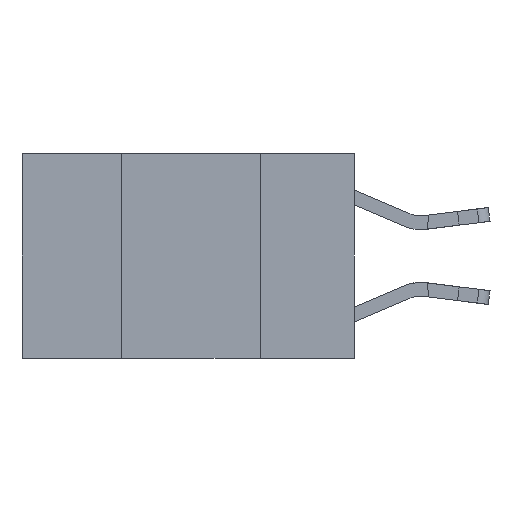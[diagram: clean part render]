
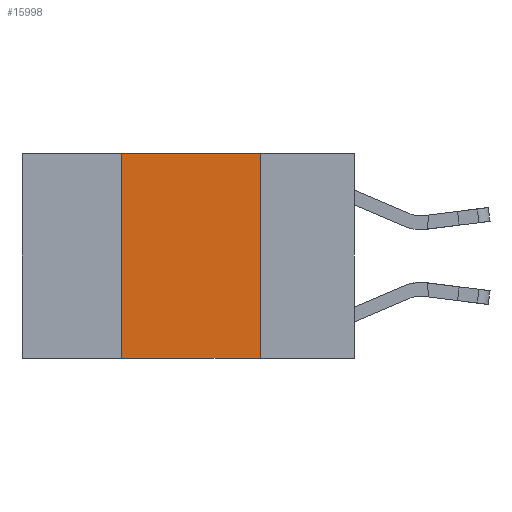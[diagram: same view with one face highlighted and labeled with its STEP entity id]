
A CAD part, left-side view. The second image highlights one B-rep face of the part: STEP entity #15998.
In plain terms, the highlighted planar face has unit normal (-1, 0, 0).
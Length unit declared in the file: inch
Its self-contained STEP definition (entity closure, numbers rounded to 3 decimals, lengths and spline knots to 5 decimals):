
#280 = EDGE_CURVE ( 'NONE', #7859, #16277, #9173, .T. ) ;
#2634 = CARTESIAN_POINT ( 'NONE',  ( 0., 0.42, -0.37 ) ) ;
#3594 = LINE ( 'NONE', #17894, #19074 ) ;
#4915 = LINE ( 'NONE', #13731, #21497 ) ;
#5844 = CARTESIAN_POINT ( 'NONE',  ( 0., 0.6, -0.37 ) ) ;
#5894 = EDGE_CURVE ( 'NONE', #19968, #14642, #3594, .T. ) ;
#7270 = FACE_OUTER_BOUND ( 'NONE', #21542, .T. ) ;
#7387 = ORIENTED_EDGE ( 'NONE', *, *, #16725, .F. ) ;
#7682 = DIRECTION ( 'NONE',  ( 0., -1., 0. ) ) ;
#7859 = VERTEX_POINT ( 'NONE', #2634 ) ;
#8364 = ORIENTED_EDGE ( 'NONE', *, *, #5894, .F. ) ;
#8982 = CARTESIAN_POINT ( 'NONE',  ( 0., 0.17, 0. ) ) ;
#9112 = VECTOR ( 'NONE', #17543, 39.37008 ) ;
#9173 = LINE ( 'NONE', #5844, #22106 ) ;
#10591 = DIRECTION ( 'NONE',  ( 1., 0., 0. ) ) ;
#11042 = DIRECTION ( 'NONE',  ( 0., 0., -1. ) ) ;
#11798 = DIRECTION ( 'NONE',  ( 0., 0., -1. ) ) ;
#13731 = CARTESIAN_POINT ( 'NONE',  ( 0., 0.17, 0. ) ) ;
#14244 = CARTESIAN_POINT ( 'NONE',  ( 0., 0.6, 0. ) ) ;
#14642 = VERTEX_POINT ( 'NONE', #8982 ) ;
#15948 = DIRECTION ( 'NONE',  ( 0., -1., 0. ) ) ;
#15998 = ADVANCED_FACE ( 'NONE', ( #7270 ), #19709, .F. ) ;
#16049 = LINE ( 'NONE', #19152, #9112 ) ;
#16277 = VERTEX_POINT ( 'NONE', #17306 ) ;
#16725 = EDGE_CURVE ( 'NONE', #14642, #16277, #4915, .T. ) ;
#17306 = CARTESIAN_POINT ( 'NONE',  ( 0., 0.17, -0.37 ) ) ;
#17543 = DIRECTION ( 'NONE',  ( 0., 0., 1. ) ) ;
#17824 = AXIS2_PLACEMENT_3D ( 'NONE', #14244, #10591, #11042 ) ;
#17894 = CARTESIAN_POINT ( 'NONE',  ( 0., 0.6, 0. ) ) ;
#18685 = ORIENTED_EDGE ( 'NONE', *, *, #280, .T. ) ;
#18710 = ORIENTED_EDGE ( 'NONE', *, *, #21850, .F. ) ;
#19074 = VECTOR ( 'NONE', #15948, 39.37008 ) ;
#19152 = CARTESIAN_POINT ( 'NONE',  ( 0., 0.42, 0. ) ) ;
#19709 = PLANE ( 'NONE',  #17824 ) ;
#19968 = VERTEX_POINT ( 'NONE', #22168 ) ;
#21497 = VECTOR ( 'NONE', #11798, 39.37008 ) ;
#21542 = EDGE_LOOP ( 'NONE', ( #7387, #8364, #18710, #18685 ) ) ;
#21850 = EDGE_CURVE ( 'NONE', #7859, #19968, #16049, .T. ) ;
#22106 = VECTOR ( 'NONE', #7682, 39.37008 ) ;
#22168 = CARTESIAN_POINT ( 'NONE',  ( 0., 0.42, 0. ) ) ;
